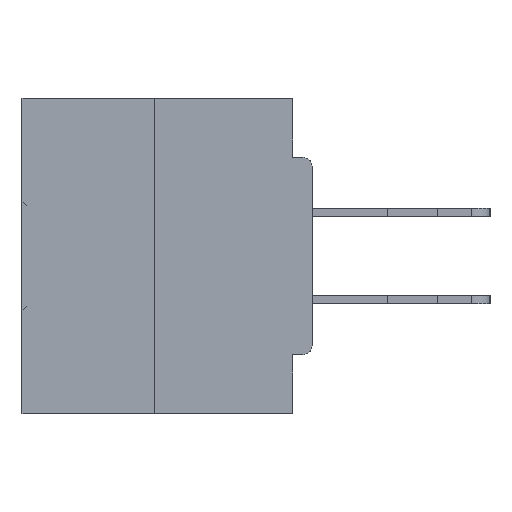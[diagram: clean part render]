
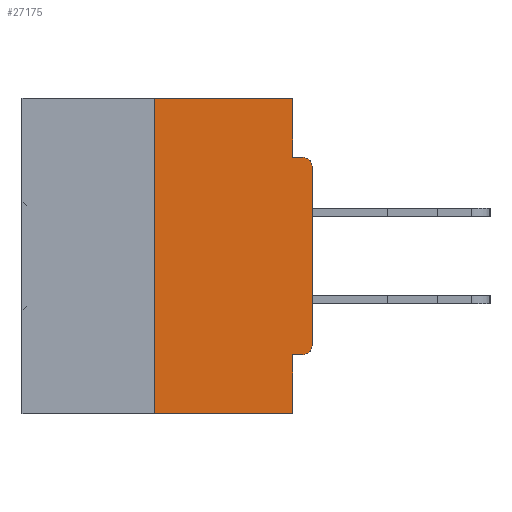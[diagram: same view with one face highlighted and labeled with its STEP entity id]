
A CAD part, left-side view. The second image highlights one B-rep face of the part: STEP entity #27175.
In plain terms, the highlighted planar face has unit normal (-1, 0, 0).
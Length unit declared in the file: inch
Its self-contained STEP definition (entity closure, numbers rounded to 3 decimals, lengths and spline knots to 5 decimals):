
#66 = DIRECTION ( 'NONE',  ( -1., 0., 0. ) ) ;
#560 = DIRECTION ( 'NONE',  ( 0., 0., -1. ) ) ;
#1107 = CARTESIAN_POINT ( 'NONE',  ( 0., 0.031, -0.5 ) ) ;
#1794 = VERTEX_POINT ( 'NONE', #5096 ) ;
#3236 = EDGE_CURVE ( 'NONE', #10105, #8497, #23408, .T. ) ;
#3572 = CARTESIAN_POINT ( 'NONE',  ( 0., 0., -0.0935 ) ) ;
#4329 = EDGE_CURVE ( 'NONE', #33088, #29565, #27974, .T. ) ;
#5096 = CARTESIAN_POINT ( 'NONE',  ( 0., 0.031, -0.0935 ) ) ;
#5137 = EDGE_CURVE ( 'NONE', #45616, #10105, #6516, .T. ) ;
#5190 = DIRECTION ( 'NONE',  ( 0., -1., 0. ) ) ;
#5441 = VERTEX_POINT ( 'NONE', #40856 ) ;
#5484 = FACE_OUTER_BOUND ( 'NONE', #45803, .T. ) ;
#6016 = EDGE_CURVE ( 'NONE', #45616, #21678, #10862, .T. ) ;
#6342 = VECTOR ( 'NONE', #24661, 39.37008 ) ;
#6516 = LINE ( 'NONE', #16705, #42774 ) ;
#6749 = DIRECTION ( 'NONE',  ( 0., 0., 1. ) ) ;
#7211 = ORIENTED_EDGE ( 'NONE', *, *, #34051, .F. ) ;
#7944 = ORIENTED_EDGE ( 'NONE', *, *, #6016, .T. ) ;
#8072 = DIRECTION ( 'NONE',  ( 0., 0., -1. ) ) ;
#8160 = CARTESIAN_POINT ( 'NONE',  ( 0., 0.031, 0. ) ) ;
#8497 = VERTEX_POINT ( 'NONE', #43375 ) ;
#9514 = ORIENTED_EDGE ( 'NONE', *, *, #22838, .F. ) ;
#9641 = ORIENTED_EDGE ( 'NONE', *, *, #3236, .F. ) ;
#9727 = CARTESIAN_POINT ( 'NONE',  ( 0., 0., -0.3915 ) ) ;
#9776 = ORIENTED_EDGE ( 'NONE', *, *, #46461, .T. ) ;
#10105 = VERTEX_POINT ( 'NONE', #27431 ) ;
#10862 = CIRCLE ( 'NONE', #45823, 0.015 ) ;
#12575 = CARTESIAN_POINT ( 'NONE',  ( 0., 0.015, -0.3915 ) ) ;
#14328 = VECTOR ( 'NONE', #18019, 39.37008 ) ;
#14815 = EDGE_CURVE ( 'NONE', #29565, #18290, #41708, .T. ) ;
#14934 = DIRECTION ( 'NONE',  ( 0., -1., 0. ) ) ;
#15010 = CARTESIAN_POINT ( 'NONE',  ( 0., 0.25, 0. ) ) ;
#16589 = CIRCLE ( 'NONE', #19596, 0.015 ) ;
#16705 = CARTESIAN_POINT ( 'NONE',  ( 0., 0., -0.4065 ) ) ;
#17632 = LINE ( 'NONE', #42326, #40027 ) ;
#17725 = ORIENTED_EDGE ( 'NONE', *, *, #46574, .T. ) ;
#17800 = CARTESIAN_POINT ( 'NONE',  ( 0., 0.46, -0.5 ) ) ;
#18019 = DIRECTION ( 'NONE',  ( 0., -1., 0. ) ) ;
#18182 = VECTOR ( 'NONE', #560, 39.37008 ) ;
#18290 = VERTEX_POINT ( 'NONE', #26193 ) ;
#19596 = AXIS2_PLACEMENT_3D ( 'NONE', #40784, #66, #8072 ) ;
#19887 = CARTESIAN_POINT ( 'NONE',  ( 0., 0.46, 0. ) ) ;
#19922 = DIRECTION ( 'NONE',  ( -1., 0., 0. ) ) ;
#20037 = VECTOR ( 'NONE', #14934, 39.37008 ) ;
#20747 = ORIENTED_EDGE ( 'NONE', *, *, #14815, .F. ) ;
#20985 = DIRECTION ( 'NONE',  ( 0., 1., 0. ) ) ;
#21559 = CARTESIAN_POINT ( 'NONE',  ( 0., 0.015, -0.4065 ) ) ;
#21678 = VERTEX_POINT ( 'NONE', #9727 ) ;
#22194 = VECTOR ( 'NONE', #5190, 39.37008 ) ;
#22838 = EDGE_CURVE ( 'NONE', #18290, #1794, #43975, .T. ) ;
#23172 = DIRECTION ( 'NONE',  ( 0., 0., -1. ) ) ;
#23408 = LINE ( 'NONE', #1107, #41824 ) ;
#23993 = ORIENTED_EDGE ( 'NONE', *, *, #39882, .T. ) ;
#24661 = DIRECTION ( 'NONE',  ( 0., 0., 1. ) ) ;
#26193 = CARTESIAN_POINT ( 'NONE',  ( 0., 0.031, 0. ) ) ;
#27175 = ADVANCED_FACE ( 'NONE', ( #5484 ), #41761, .F. ) ;
#27431 = CARTESIAN_POINT ( 'NONE',  ( 0., 0.031, -0.4065 ) ) ;
#27974 = LINE ( 'NONE', #42910, #6342 ) ;
#28247 = VERTEX_POINT ( 'NONE', #44580 ) ;
#28742 = ORIENTED_EDGE ( 'NONE', *, *, #5137, .F. ) ;
#29565 = VERTEX_POINT ( 'NONE', #15010 ) ;
#29623 = LINE ( 'NONE', #3572, #14328 ) ;
#31307 = DIRECTION ( 'NONE',  ( 0., 0., -1. ) ) ;
#32190 = CARTESIAN_POINT ( 'NONE',  ( 0., 0.25, -0.5 ) ) ;
#32950 = LINE ( 'NONE', #17800, #20037 ) ;
#33088 = VERTEX_POINT ( 'NONE', #32190 ) ;
#34051 = EDGE_CURVE ( 'NONE', #1794, #5441, #29623, .T. ) ;
#38659 = CARTESIAN_POINT ( 'NONE',  ( 0., 0.46, 0. ) ) ;
#38991 = AXIS2_PLACEMENT_3D ( 'NONE', #38659, #46018, #31307 ) ;
#39882 = EDGE_CURVE ( 'NONE', #33088, #8497, #32950, .T. ) ;
#40027 = VECTOR ( 'NONE', #6749, 39.37008 ) ;
#40784 = CARTESIAN_POINT ( 'NONE',  ( 0., 0.015, -0.1085 ) ) ;
#40856 = CARTESIAN_POINT ( 'NONE',  ( 0., 0.015, -0.0935 ) ) ;
#41277 = ORIENTED_EDGE ( 'NONE', *, *, #4329, .F. ) ;
#41708 = LINE ( 'NONE', #19887, #22194 ) ;
#41761 = PLANE ( 'NONE',  #38991 ) ;
#41824 = VECTOR ( 'NONE', #23172, 39.37008 ) ;
#42326 = CARTESIAN_POINT ( 'NONE',  ( 0., 0., 0. ) ) ;
#42774 = VECTOR ( 'NONE', #20985, 39.37008 ) ;
#42910 = CARTESIAN_POINT ( 'NONE',  ( 0., 0.25, 0. ) ) ;
#43089 = DIRECTION ( 'NONE',  ( 0., 0., -1. ) ) ;
#43375 = CARTESIAN_POINT ( 'NONE',  ( 0., 0.031, -0.5 ) ) ;
#43975 = LINE ( 'NONE', #8160, #18182 ) ;
#44580 = CARTESIAN_POINT ( 'NONE',  ( 0., 0., -0.1085 ) ) ;
#45616 = VERTEX_POINT ( 'NONE', #21559 ) ;
#45803 = EDGE_LOOP ( 'NONE', ( #20747, #41277, #23993, #9641, #28742, #7944, #9776, #17725, #7211, #9514 ) ) ;
#45823 = AXIS2_PLACEMENT_3D ( 'NONE', #12575, #19922, #43089 ) ;
#46018 = DIRECTION ( 'NONE',  ( 1., 0., 0. ) ) ;
#46461 = EDGE_CURVE ( 'NONE', #21678, #28247, #17632, .T. ) ;
#46574 = EDGE_CURVE ( 'NONE', #28247, #5441, #16589, .T. ) ;
